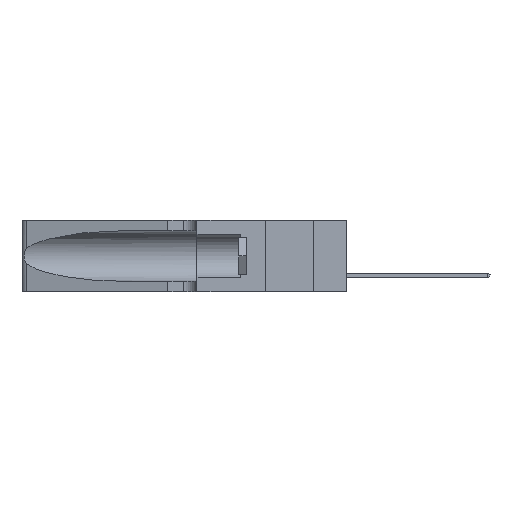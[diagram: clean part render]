
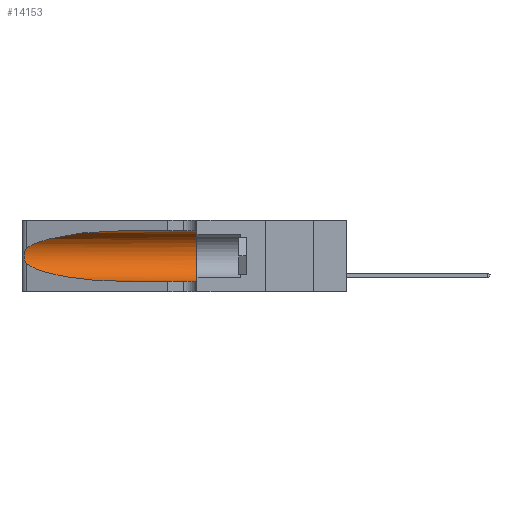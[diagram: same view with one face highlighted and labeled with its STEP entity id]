
A CAD part, left-side view. The second image highlights one B-rep face of the part: STEP entity #14153.
In plain terms, the highlighted cylindrical face has radius 3.308 mm (diameter 6.617 mm), a partial arc.
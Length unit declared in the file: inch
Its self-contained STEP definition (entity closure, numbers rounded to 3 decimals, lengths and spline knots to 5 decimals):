
#418 = CARTESIAN_POINT ( 'NONE',  ( 0.18966, 0.96281, 0.05475 ) ) ;
#576 = ORIENTED_EDGE ( 'NONE', *, *, #36331, .F. ) ;
#1412 = CARTESIAN_POINT ( 'NONE',  ( 0.26017, 1.23833, 0.17102 ) ) ;
#1765 = LINE ( 'NONE', #6571, #24269 ) ;
#2838 = ORIENTED_EDGE ( 'NONE', *, *, #19254, .T. ) ;
#4529 = CARTESIAN_POINT ( 'NONE',  ( 0.25487, 1.22718, 0.22369 ) ) ;
#5365 = CARTESIAN_POINT ( 'NONE',  ( 0.25487, 1.22718, 0.22369 ) ) ;
#5865 = CARTESIAN_POINT ( 'NONE',  ( 0.25487, 1.22718, 0.22369 ) ) ;
#6388 = CIRCLE ( 'NONE', #8028, 0.13025 ) ;
#6571 = CARTESIAN_POINT ( 'NONE',  ( 0.1305, 1.61858, 0.31525 ) ) ;
#7146 = EDGE_CURVE ( 'NONE', #11134, #41542, #6388, .T. ) ;
#7850 = CARTESIAN_POINT ( 'NONE',  ( 0.25787, 1.23484, 0.2124 ) ) ;
#7950 = ORIENTED_EDGE ( 'NONE', *, *, #8453, .T. ) ;
#8004 = CARTESIAN_POINT ( 'NONE',  ( 0.1305, 0.72297, 0.05475 ) ) ;
#8028 = AXIS2_PLACEMENT_3D ( 'NONE', #15448, #34171, #22820 ) ;
#8307 = CARTESIAN_POINT ( 'NONE',  ( 0.25639, 1.23186, 0.15144 ) ) ;
#8453 = EDGE_CURVE ( 'NONE', #36192, #41542, #40757, .T. ) ;
#10058 = DIRECTION ( 'NONE',  ( 0., 0., -1. ) ) ;
#11134 = VERTEX_POINT ( 'NONE', #46128 ) ;
#11559 = CARTESIAN_POINT ( 'NONE',  ( 0.25856, 1.23593, 0.16098 ) ) ;
#12074 = EDGE_CURVE ( 'NONE', #38402, #19670, #41860, .T. ) ;
#12089 = CARTESIAN_POINT ( 'NONE',  ( 0.25487, 1.22718, 0.14631 ) ) ;
#14153 = ADVANCED_FACE ( 'NONE', ( #18471 ), #15957, .F. ) ;
#14796 = B_SPLINE_CURVE_WITH_KNOTS ( 'NONE', 3,
 ( #5365, #19544, #31286, #7850, #39020, #19859, #39989, #47334, #1412, #11559, #38096, #8307, #43267, #32725 ),
 .UNSPECIFIED., .F., .F.,
 ( 4, 2, 2, 2, 2, 2, 4 ),
 ( 0., 0.00027, 0.00053, 0.00107, 0.0016, 0.00187, 0.00214 ),
 .UNSPECIFIED. ) ;
#15448 = CARTESIAN_POINT ( 'NONE',  ( 0.1305, 0.35, 0.185 ) ) ;
#15957 = CYLINDRICAL_SURFACE ( 'NONE', #45058, 0.13025 ) ;
#17764 = DIRECTION ( 'NONE',  ( 0., -1., 0. ) ) ;
#18471 = FACE_OUTER_BOUND ( 'NONE', #29652, .T. ) ;
#19254 = EDGE_CURVE ( 'NONE', #19670, #26901, #14796, .T. ) ;
#19544 = CARTESIAN_POINT ( 'NONE',  ( 0.25555, 1.22994, 0.2215 ) ) ;
#19670 = VERTEX_POINT ( 'NONE', #5865 ) ;
#19838 = CARTESIAN_POINT ( 'NONE',  ( 0.2373, 1.15595, 0.28018 ) ) ;
#19859 = CARTESIAN_POINT ( 'NONE',  ( 0.26018, 1.23835, 0.19895 ) ) ;
#19871 = CARTESIAN_POINT ( 'NONE',  ( 0.2373, 1.15595, 0.08982 ) ) ;
#22820 = DIRECTION ( 'NONE',  ( 0., 0., 1. ) ) ;
#24269 = VECTOR ( 'NONE', #32261, 39.37008 ) ;
#25210 = CARTESIAN_POINT ( 'NONE',  ( 0.25487, 1.22718, 0.14631 ) ) ;
#26710 = DIRECTION ( 'NONE',  ( 0., -1., 0. ) ) ;
#26901 = VERTEX_POINT ( 'NONE', #25210 ) ;
#27938 = CARTESIAN_POINT ( 'NONE',  ( 0.1305, 0.72297, 0.05475 ) ) ;
#29652 = EDGE_LOOP ( 'NONE', ( #32551, #2838, #38593, #7950, #45764, #576 ) ) ;
#31286 = CARTESIAN_POINT ( 'NONE',  ( 0.25639, 1.23184, 0.21858 ) ) ;
#32261 = DIRECTION ( 'NONE',  ( 0., -1., 0. ) ) ;
#32551 = ORIENTED_EDGE ( 'NONE', *, *, #12074, .T. ) ;
#32725 = CARTESIAN_POINT ( 'NONE',  ( 0.25487, 1.22718, 0.14631 ) ) ;
#34171 = DIRECTION ( 'NONE',  ( 0., 1., 0. ) ) ;
#36192 = VERTEX_POINT ( 'NONE', #27938 ) ;
#36331 = EDGE_CURVE ( 'NONE', #38402, #11134, #1765, .T. ) ;
#36686 = CARTESIAN_POINT ( 'NONE',  ( 0.1305, 0.35, 0.05475 ) ) ;
#38096 = CARTESIAN_POINT ( 'NONE',  ( 0.25789, 1.23486, 0.15765 ) ) ;
#38402 = VERTEX_POINT ( 'NONE', #44097 ) ;
#38593 = ORIENTED_EDGE ( 'NONE', *, *, #49109, .T. ) ;
#39020 = CARTESIAN_POINT ( 'NONE',  ( 0.25854, 1.2359, 0.20912 ) ) ;
#39479 = CARTESIAN_POINT ( 'NONE',  ( 0.1305, 0.72297, 0.31525 ) ) ;
#39989 = CARTESIAN_POINT ( 'NONE',  ( 0.26075, 1.23896, 0.19203 ) ) ;
#40757 = LINE ( 'NONE', #47236, #43764 ) ;
#41542 = VERTEX_POINT ( 'NONE', #36686 ) ;
#41860 =( BOUNDED_CURVE ( )  B_SPLINE_CURVE ( 3, ( #39479, #46913, #19838, #4529 ),
 .UNSPECIFIED., .F., .T. ) 
 B_SPLINE_CURVE_WITH_KNOTS ( ( 4, 4 ),
 ( 1.5708, 2.84003 ),
 .UNSPECIFIED. ) 
 CURVE ( )  GEOMETRIC_REPRESENTATION_ITEM ( )  RATIONAL_B_SPLINE_CURVE ( ( 1., 0.87, 0.87, 1. ) ) 
 REPRESENTATION_ITEM ( '' )  );
#43267 = CARTESIAN_POINT ( 'NONE',  ( 0.25555, 1.22993, 0.14849 ) ) ;
#43764 = VECTOR ( 'NONE', #17764, 39.37008 ) ;
#44097 = CARTESIAN_POINT ( 'NONE',  ( 0.1305, 0.72297, 0.31525 ) ) ;
#45058 = AXIS2_PLACEMENT_3D ( 'NONE', #49994, #26710, #10058 ) ;
#45764 = ORIENTED_EDGE ( 'NONE', *, *, #7146, .F. ) ;
#46128 = CARTESIAN_POINT ( 'NONE',  ( 0.1305, 0.35, 0.31525 ) ) ;
#46913 = CARTESIAN_POINT ( 'NONE',  ( 0.18966, 0.96281, 0.31525 ) ) ;
#47236 = CARTESIAN_POINT ( 'NONE',  ( 0.1305, 1.61858, 0.05475 ) ) ;
#47334 = CARTESIAN_POINT ( 'NONE',  ( 0.26075, 1.23896, 0.178 ) ) ;
#49053 =( BOUNDED_CURVE ( )  B_SPLINE_CURVE ( 3, ( #12089, #19871, #418, #8004 ),
 .UNSPECIFIED., .F., .T. ) 
 B_SPLINE_CURVE_WITH_KNOTS ( ( 4, 4 ),
 ( 3.44316, 4.71239 ),
 .UNSPECIFIED. ) 
 CURVE ( )  GEOMETRIC_REPRESENTATION_ITEM ( )  RATIONAL_B_SPLINE_CURVE ( ( 1., 0.87, 0.87, 1. ) ) 
 REPRESENTATION_ITEM ( '' )  );
#49109 = EDGE_CURVE ( 'NONE', #26901, #36192, #49053, .T. ) ;
#49994 = CARTESIAN_POINT ( 'NONE',  ( 0.1305, 1.61858, 0.185 ) ) ;
